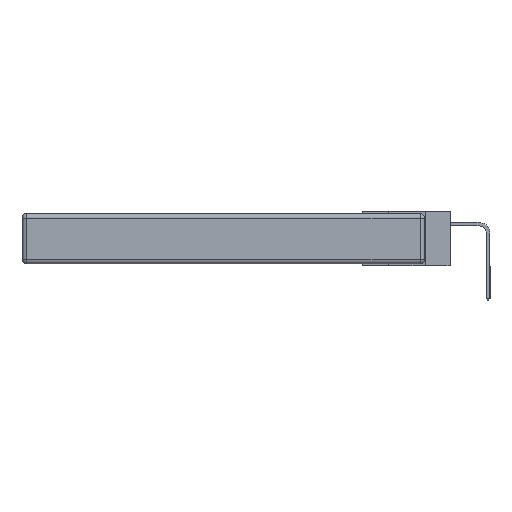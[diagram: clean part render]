
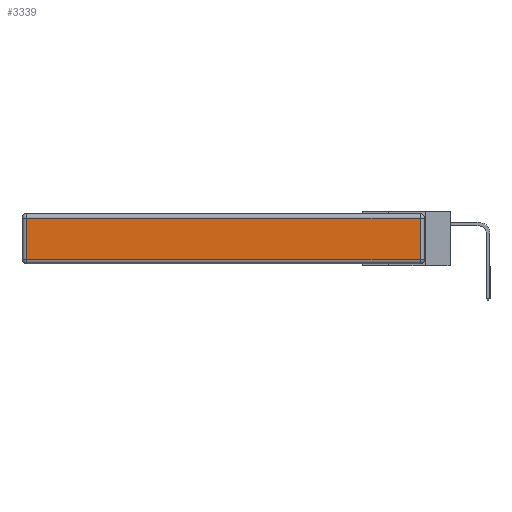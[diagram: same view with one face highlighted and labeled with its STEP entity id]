
A CAD part, left-side view. The second image highlights one B-rep face of the part: STEP entity #3339.
In plain terms, the highlighted planar face has unit normal (-1, 0, 0).
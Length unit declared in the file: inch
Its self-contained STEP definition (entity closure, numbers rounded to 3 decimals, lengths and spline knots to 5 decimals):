
#1231 = VECTOR ( 'NONE', #8936, 39.37008 ) ;
#1363 = VERTEX_POINT ( 'NONE', #2938 ) ;
#1397 = CARTESIAN_POINT ( 'NONE',  ( 0., 2.72, -0.313 ) ) ;
#1942 = ORIENTED_EDGE ( 'NONE', *, *, #13804, .T. ) ;
#2173 = VERTEX_POINT ( 'NONE', #6376 ) ;
#2358 = LINE ( 'NONE', #8094, #13180 ) ;
#2938 = CARTESIAN_POINT ( 'NONE',  ( 0., 2.72, -0.03 ) ) ;
#3339 = ADVANCED_FACE ( 'NONE', ( #12468 ), #12050, .T. ) ;
#4608 = EDGE_CURVE ( 'NONE', #10508, #2173, #10323, .T. ) ;
#4892 = EDGE_CURVE ( 'NONE', #2173, #13651, #6225, .T. ) ;
#5652 = ORIENTED_EDGE ( 'NONE', *, *, #13201, .T. ) ;
#5655 = DIRECTION ( 'NONE',  ( 0., 0., -1. ) ) ;
#5833 = ORIENTED_EDGE ( 'NONE', *, *, #4608, .T. ) ;
#6225 = LINE ( 'NONE', #7762, #15173 ) ;
#6376 = CARTESIAN_POINT ( 'NONE',  ( 0., 0.03, -0.313 ) ) ;
#6759 = DIRECTION ( 'NONE',  ( 0., 0., 1. ) ) ;
#7762 = CARTESIAN_POINT ( 'NONE',  ( 0., 0.03, -0.343 ) ) ;
#8094 = CARTESIAN_POINT ( 'NONE',  ( 0., 2.72, -0.343 ) ) ;
#8449 = ORIENTED_EDGE ( 'NONE', *, *, #4892, .T. ) ;
#8460 = DIRECTION ( 'NONE',  ( 0., -1., 0. ) ) ;
#8613 = CARTESIAN_POINT ( 'NONE',  ( 0., 0., -0.313 ) ) ;
#8936 = DIRECTION ( 'NONE',  ( 0., 1., 0. ) ) ;
#9237 = EDGE_LOOP ( 'NONE', ( #5833, #8449, #1942, #5652 ) ) ;
#9466 = DIRECTION ( 'NONE',  ( -1., 0., 0. ) ) ;
#9827 = LINE ( 'NONE', #11418, #1231 ) ;
#10323 = LINE ( 'NONE', #8613, #13473 ) ;
#10508 = VERTEX_POINT ( 'NONE', #1397 ) ;
#10862 = CARTESIAN_POINT ( 'NONE',  ( 0., 0.03, -0.03 ) ) ;
#11418 = CARTESIAN_POINT ( 'NONE',  ( 0., 2.75, -0.03 ) ) ;
#11701 = AXIS2_PLACEMENT_3D ( 'NONE', #14365, #9466, #14215 ) ;
#12050 = PLANE ( 'NONE',  #11701 ) ;
#12468 = FACE_OUTER_BOUND ( 'NONE', #9237, .T. ) ;
#13180 = VECTOR ( 'NONE', #5655, 39.37008 ) ;
#13201 = EDGE_CURVE ( 'NONE', #1363, #10508, #2358, .T. ) ;
#13473 = VECTOR ( 'NONE', #8460, 39.37008 ) ;
#13651 = VERTEX_POINT ( 'NONE', #10862 ) ;
#13804 = EDGE_CURVE ( 'NONE', #13651, #1363, #9827, .T. ) ;
#14215 = DIRECTION ( 'NONE',  ( 0., 0., 1. ) ) ;
#14365 = CARTESIAN_POINT ( 'NONE',  ( 0., 0., -0.343 ) ) ;
#15173 = VECTOR ( 'NONE', #6759, 39.37008 ) ;
